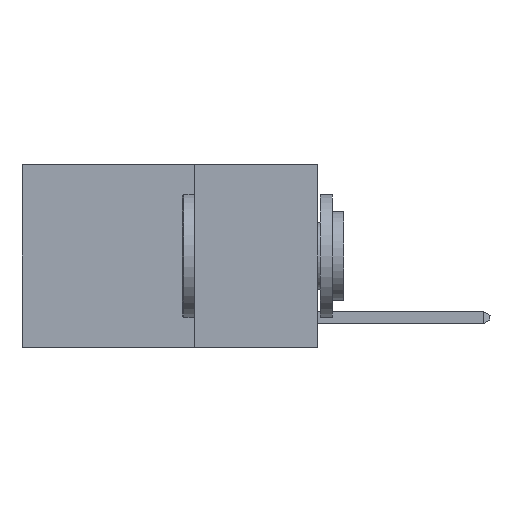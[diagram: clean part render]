
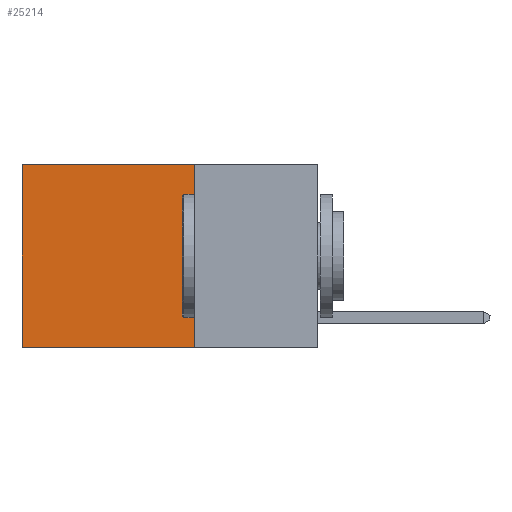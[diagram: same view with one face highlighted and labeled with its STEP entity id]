
A CAD part, left-side view. The second image highlights one B-rep face of the part: STEP entity #25214.
In plain terms, the highlighted planar face has unit normal (-1, 0, 0).
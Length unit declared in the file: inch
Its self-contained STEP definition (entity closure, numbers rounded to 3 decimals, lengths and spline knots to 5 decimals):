
#1418 = LINE ( 'NONE', #1812, #14726 ) ;
#1667 = ORIENTED_EDGE ( 'NONE', *, *, #25397, .F. ) ;
#1812 = CARTESIAN_POINT ( 'NONE',  ( 0.2625, 0.25, 0. ) ) ;
#2002 = LINE ( 'NONE', #26006, #21708 ) ;
#2198 = VECTOR ( 'NONE', #11325, 39.37008 ) ;
#2252 = CARTESIAN_POINT ( 'NONE',  ( 0.2625, 0.6, -0.37 ) ) ;
#2446 = CARTESIAN_POINT ( 'NONE',  ( 0.2625, 0.25, 0. ) ) ;
#2730 = LINE ( 'NONE', #25008, #15368 ) ;
#2874 = ORIENTED_EDGE ( 'NONE', *, *, #8862, .F. ) ;
#3255 = CARTESIAN_POINT ( 'NONE',  ( 0.2625, 0.25, 0. ) ) ;
#5235 = DIRECTION ( 'NONE',  ( 0., 0., -1. ) ) ;
#6661 = CARTESIAN_POINT ( 'NONE',  ( 0.2625, 0.6, 0. ) ) ;
#7840 = CARTESIAN_POINT ( 'NONE',  ( 0.2625, 0.25, 0. ) ) ;
#8862 = EDGE_CURVE ( 'NONE', #21155, #9112, #1418, .T. ) ;
#9112 = VERTEX_POINT ( 'NONE', #10047 ) ;
#9384 = DIRECTION ( 'NONE',  ( 0., 0., -1. ) ) ;
#10047 = CARTESIAN_POINT ( 'NONE',  ( 0.2625, 0.25, -0.37 ) ) ;
#10269 = DIRECTION ( 'NONE',  ( 0., 0., -1. ) ) ;
#10824 = LINE ( 'NONE', #3255, #2198 ) ;
#11325 = DIRECTION ( 'NONE',  ( 0., 1., 0. ) ) ;
#11366 = VERTEX_POINT ( 'NONE', #2252 ) ;
#13536 = VERTEX_POINT ( 'NONE', #6661 ) ;
#14092 = AXIS2_PLACEMENT_3D ( 'NONE', #2446, #25951, #10269 ) ;
#14234 = FACE_OUTER_BOUND ( 'NONE', #22876, .T. ) ;
#14491 = PLANE ( 'NONE',  #14092 ) ;
#14566 = EDGE_CURVE ( 'NONE', #21155, #13536, #10824, .T. ) ;
#14726 = VECTOR ( 'NONE', #9384, 39.37008 ) ;
#15368 = VECTOR ( 'NONE', #5235, 39.37008 ) ;
#15906 = ORIENTED_EDGE ( 'NONE', *, *, #14566, .T. ) ;
#17554 = ORIENTED_EDGE ( 'NONE', *, *, #25843, .T. ) ;
#21155 = VERTEX_POINT ( 'NONE', #7840 ) ;
#21708 = VECTOR ( 'NONE', #25377, 39.37008 ) ;
#22876 = EDGE_LOOP ( 'NONE', ( #17554, #1667, #2874, #15906 ) ) ;
#25008 = CARTESIAN_POINT ( 'NONE',  ( 0.2625, 0.6, 0. ) ) ;
#25214 = ADVANCED_FACE ( 'NONE', ( #14234 ), #14491, .F. ) ;
#25377 = DIRECTION ( 'NONE',  ( 0., 1., 0. ) ) ;
#25397 = EDGE_CURVE ( 'NONE', #9112, #11366, #2002, .T. ) ;
#25843 = EDGE_CURVE ( 'NONE', #13536, #11366, #2730, .T. ) ;
#25951 = DIRECTION ( 'NONE',  ( 1., 0., 0. ) ) ;
#26006 = CARTESIAN_POINT ( 'NONE',  ( 0.2625, 0.25, -0.37 ) ) ;
